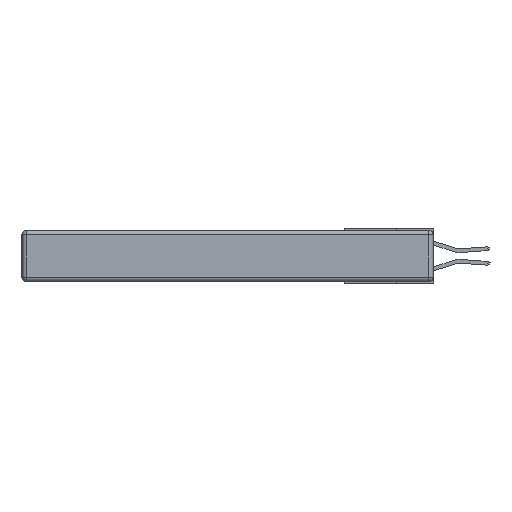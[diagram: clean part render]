
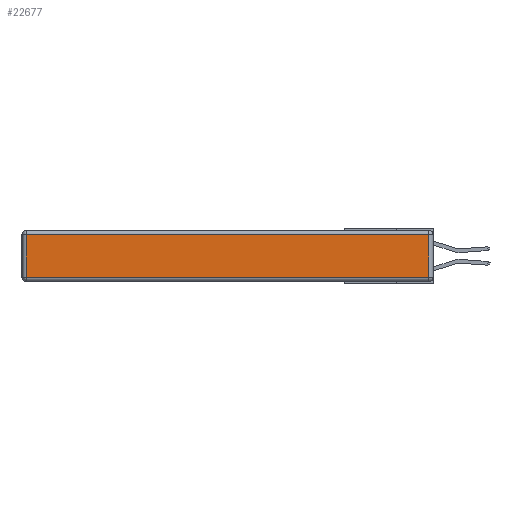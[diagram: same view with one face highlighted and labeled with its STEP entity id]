
A CAD part, left-side view. The second image highlights one B-rep face of the part: STEP entity #22677.
In plain terms, the highlighted planar face has unit normal (-1, 0, 0).
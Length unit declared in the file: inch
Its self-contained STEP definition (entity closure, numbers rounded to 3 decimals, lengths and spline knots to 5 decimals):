
#1259 = VERTEX_POINT ( 'NONE', #5944 ) ;
#1670 = EDGE_CURVE ( 'NONE', #13433, #1259, #28496, .T. ) ;
#2177 = VECTOR ( 'NONE', #30436, 39.37008 ) ;
#5593 = EDGE_CURVE ( 'NONE', #9816, #27832, #30419, .T. ) ;
#5944 = CARTESIAN_POINT ( 'NONE',  ( 0., 0.03, -0.313 ) ) ;
#8535 = ORIENTED_EDGE ( 'NONE', *, *, #1670, .T. ) ;
#8713 = CARTESIAN_POINT ( 'NONE',  ( 0., 0., -0.343 ) ) ;
#9011 = ORIENTED_EDGE ( 'NONE', *, *, #11729, .T. ) ;
#9602 = DIRECTION ( 'NONE',  ( 0., 1., 0. ) ) ;
#9816 = VERTEX_POINT ( 'NONE', #25697 ) ;
#10571 = CARTESIAN_POINT ( 'NONE',  ( 0., 0.03, -0.343 ) ) ;
#11729 = EDGE_CURVE ( 'NONE', #1259, #9816, #21026, .T. ) ;
#12047 = EDGE_LOOP ( 'NONE', ( #8535, #9011, #21434, #32187 ) ) ;
#12177 = AXIS2_PLACEMENT_3D ( 'NONE', #8713, #21462, #21577 ) ;
#12241 = PLANE ( 'NONE',  #12177 ) ;
#13433 = VERTEX_POINT ( 'NONE', #14937 ) ;
#14937 = CARTESIAN_POINT ( 'NONE',  ( 0., 2.72, -0.313 ) ) ;
#14995 = VECTOR ( 'NONE', #9602, 39.37008 ) ;
#15081 = CARTESIAN_POINT ( 'NONE',  ( 0., 2.75, -0.03 ) ) ;
#15649 = VECTOR ( 'NONE', #27969, 39.37008 ) ;
#16164 = VECTOR ( 'NONE', #34861, 39.37008 ) ;
#18023 = FACE_OUTER_BOUND ( 'NONE', #12047, .T. ) ;
#18919 = CARTESIAN_POINT ( 'NONE',  ( 0., 0., -0.313 ) ) ;
#21026 = LINE ( 'NONE', #10571, #2177 ) ;
#21434 = ORIENTED_EDGE ( 'NONE', *, *, #5593, .T. ) ;
#21462 = DIRECTION ( 'NONE',  ( -1., 0., 0. ) ) ;
#21577 = DIRECTION ( 'NONE',  ( 0., 0., 1. ) ) ;
#22552 = CARTESIAN_POINT ( 'NONE',  ( 0., 2.72, -0.03 ) ) ;
#22677 = ADVANCED_FACE ( 'NONE', ( #18023 ), #12241, .T. ) ;
#24432 = EDGE_CURVE ( 'NONE', #27832, #13433, #27777, .T. ) ;
#25697 = CARTESIAN_POINT ( 'NONE',  ( 0., 0.03, -0.03 ) ) ;
#27777 = LINE ( 'NONE', #31164, #16164 ) ;
#27832 = VERTEX_POINT ( 'NONE', #22552 ) ;
#27969 = DIRECTION ( 'NONE',  ( 0., -1., 0. ) ) ;
#28496 = LINE ( 'NONE', #18919, #15649 ) ;
#30419 = LINE ( 'NONE', #15081, #14995 ) ;
#30436 = DIRECTION ( 'NONE',  ( 0., 0., 1. ) ) ;
#31164 = CARTESIAN_POINT ( 'NONE',  ( 0., 2.72, -0.343 ) ) ;
#32187 = ORIENTED_EDGE ( 'NONE', *, *, #24432, .T. ) ;
#34861 = DIRECTION ( 'NONE',  ( 0., 0., -1. ) ) ;
